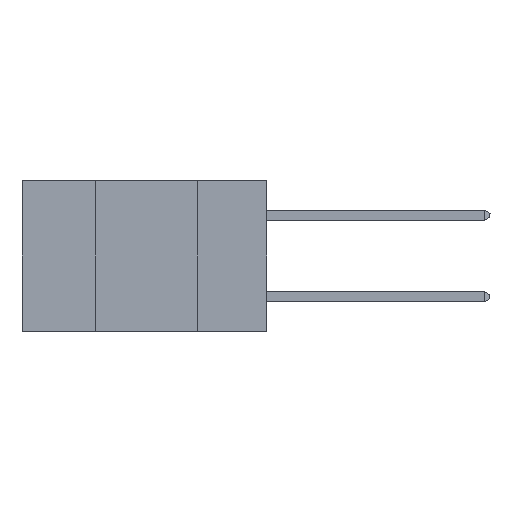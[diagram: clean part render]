
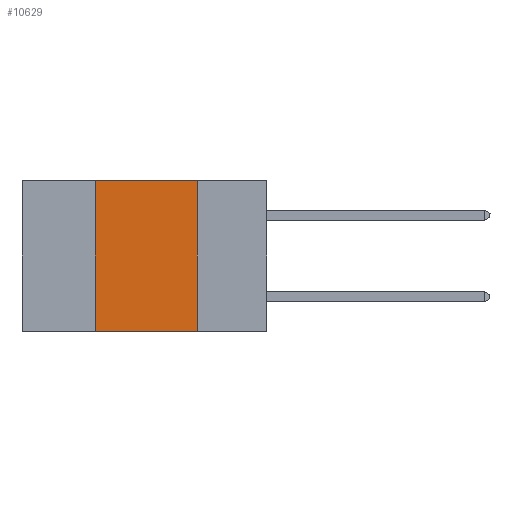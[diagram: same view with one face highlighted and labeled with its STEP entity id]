
A CAD part, left-side view. The second image highlights one B-rep face of the part: STEP entity #10629.
In plain terms, the highlighted planar face has unit normal (-1, 0, 0).
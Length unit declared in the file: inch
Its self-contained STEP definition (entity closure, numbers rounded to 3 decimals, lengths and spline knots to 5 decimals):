
#82 = EDGE_LOOP ( 'NONE', ( #9758, #25580, #11631, #6875 ) ) ;
#784 = CARTESIAN_POINT ( 'NONE',  ( 0., 0.6, -0.37 ) ) ;
#974 = LINE ( 'NONE', #11226, #17372 ) ;
#4335 = EDGE_CURVE ( 'NONE', #27837, #36834, #17857, .T. ) ;
#6450 = VERTEX_POINT ( 'NONE', #19128 ) ;
#6487 = VECTOR ( 'NONE', #26653, 39.37008 ) ;
#6875 = ORIENTED_EDGE ( 'NONE', *, *, #8105, .T. ) ;
#8105 = EDGE_CURVE ( 'NONE', #6450, #12016, #15935, .T. ) ;
#9515 = DIRECTION ( 'NONE',  ( 0., 0., -1. ) ) ;
#9758 = ORIENTED_EDGE ( 'NONE', *, *, #24655, .F. ) ;
#9771 = DIRECTION ( 'NONE',  ( 1., 0., 0. ) ) ;
#10629 = ADVANCED_FACE ( 'NONE', ( #14844 ), #26902, .F. ) ;
#10651 = CARTESIAN_POINT ( 'NONE',  ( 0., 0.17, -0.37 ) ) ;
#11226 = CARTESIAN_POINT ( 'NONE',  ( 0., 0.42, 0. ) ) ;
#11631 = ORIENTED_EDGE ( 'NONE', *, *, #31308, .F. ) ;
#12016 = VERTEX_POINT ( 'NONE', #10651 ) ;
#14177 = DIRECTION ( 'NONE',  ( 0., 0., 1. ) ) ;
#14844 = FACE_OUTER_BOUND ( 'NONE', #82, .T. ) ;
#15935 = LINE ( 'NONE', #784, #34525 ) ;
#17372 = VECTOR ( 'NONE', #14177, 39.37008 ) ;
#17656 = AXIS2_PLACEMENT_3D ( 'NONE', #18295, #9771, #9515 ) ;
#17857 = LINE ( 'NONE', #29460, #6487 ) ;
#18295 = CARTESIAN_POINT ( 'NONE',  ( 0., 0.6, 0. ) ) ;
#19128 = CARTESIAN_POINT ( 'NONE',  ( 0., 0.42, -0.37 ) ) ;
#23566 = CARTESIAN_POINT ( 'NONE',  ( 0., 0.42, 0. ) ) ;
#24594 = CARTESIAN_POINT ( 'NONE',  ( 0., 0.17, 0. ) ) ;
#24655 = EDGE_CURVE ( 'NONE', #36834, #12016, #36106, .T. ) ;
#25580 = ORIENTED_EDGE ( 'NONE', *, *, #4335, .F. ) ;
#26653 = DIRECTION ( 'NONE',  ( 0., -1., 0. ) ) ;
#26902 = PLANE ( 'NONE',  #17656 ) ;
#26947 = DIRECTION ( 'NONE',  ( 0., -1., 0. ) ) ;
#27837 = VERTEX_POINT ( 'NONE', #23566 ) ;
#29335 = VECTOR ( 'NONE', #33344, 39.37008 ) ;
#29460 = CARTESIAN_POINT ( 'NONE',  ( 0., 0.6, 0. ) ) ;
#31308 = EDGE_CURVE ( 'NONE', #6450, #27837, #974, .T. ) ;
#32085 = CARTESIAN_POINT ( 'NONE',  ( 0., 0.17, 0. ) ) ;
#33344 = DIRECTION ( 'NONE',  ( 0., 0., -1. ) ) ;
#34525 = VECTOR ( 'NONE', #26947, 39.37008 ) ;
#36106 = LINE ( 'NONE', #24594, #29335 ) ;
#36834 = VERTEX_POINT ( 'NONE', #32085 ) ;
